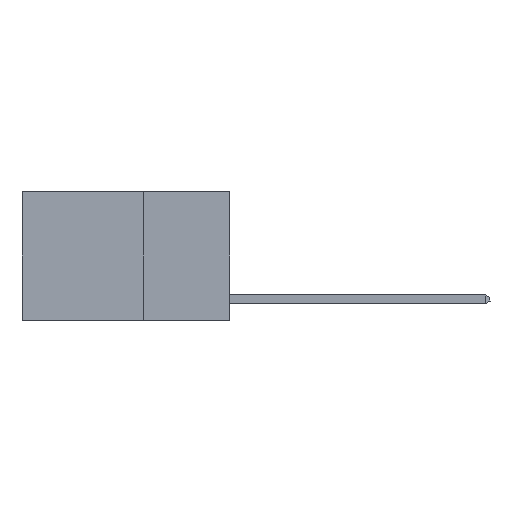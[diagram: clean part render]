
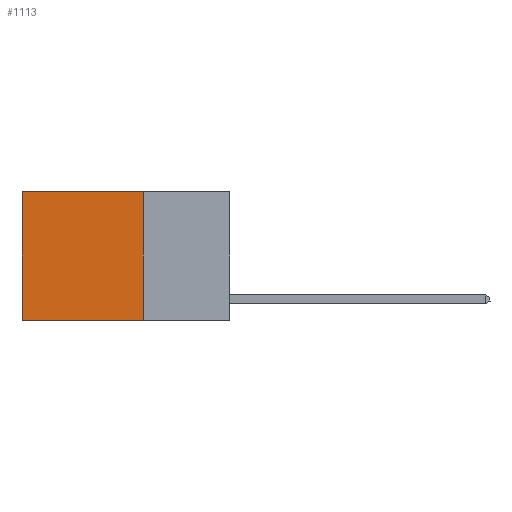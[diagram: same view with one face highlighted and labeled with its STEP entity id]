
A CAD part, left-side view. The second image highlights one B-rep face of the part: STEP entity #1113.
In plain terms, the highlighted planar face has unit normal (-1, 0, 0).
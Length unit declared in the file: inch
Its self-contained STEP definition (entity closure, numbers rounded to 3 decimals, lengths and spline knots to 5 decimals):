
#181 = DIRECTION ( 'NONE',  ( 1., 0., 0. ) ) ;
#607 = CARTESIAN_POINT ( 'NONE',  ( 0.2625, 0.25, -0.37 ) ) ;
#617 = VECTOR ( 'NONE', #15308, 39.37008 ) ;
#680 = CARTESIAN_POINT ( 'NONE',  ( 0.2625, 0.25, 0. ) ) ;
#1113 = ADVANCED_FACE ( 'NONE', ( #6181 ), #6401, .F. ) ;
#1139 = LINE ( 'NONE', #12861, #6908 ) ;
#1286 = VERTEX_POINT ( 'NONE', #11385 ) ;
#1563 = CARTESIAN_POINT ( 'NONE',  ( 0.2625, 0.6, 0. ) ) ;
#1657 = AXIS2_PLACEMENT_3D ( 'NONE', #13498, #181, #7587 ) ;
#2955 = ORIENTED_EDGE ( 'NONE', *, *, #6551, .F. ) ;
#3076 = EDGE_CURVE ( 'NONE', #11134, #11323, #7066, .T. ) ;
#3170 = VECTOR ( 'NONE', #4371, 39.37008 ) ;
#3429 = DIRECTION ( 'NONE',  ( 0., 1., 0. ) ) ;
#4371 = DIRECTION ( 'NONE',  ( 0., 0., -1. ) ) ;
#5027 = EDGE_CURVE ( 'NONE', #10386, #1286, #1139, .T. ) ;
#6181 = FACE_OUTER_BOUND ( 'NONE', #11039, .T. ) ;
#6401 = PLANE ( 'NONE',  #1657 ) ;
#6551 = EDGE_CURVE ( 'NONE', #11323, #1286, #6886, .T. ) ;
#6660 = DIRECTION ( 'NONE',  ( 0., 0., -1. ) ) ;
#6662 = ORIENTED_EDGE ( 'NONE', *, *, #3076, .F. ) ;
#6707 = ORIENTED_EDGE ( 'NONE', *, *, #10562, .T. ) ;
#6886 = LINE ( 'NONE', #7164, #10691 ) ;
#6908 = VECTOR ( 'NONE', #6660, 39.37008 ) ;
#7066 = LINE ( 'NONE', #680, #3170 ) ;
#7164 = CARTESIAN_POINT ( 'NONE',  ( 0.2625, 0.25, -0.37 ) ) ;
#7587 = DIRECTION ( 'NONE',  ( 0., 0., -1. ) ) ;
#9226 = CARTESIAN_POINT ( 'NONE',  ( 0.2625, 0.25, 0. ) ) ;
#10386 = VERTEX_POINT ( 'NONE', #1563 ) ;
#10562 = EDGE_CURVE ( 'NONE', #11134, #10386, #15433, .T. ) ;
#10691 = VECTOR ( 'NONE', #3429, 39.37008 ) ;
#11039 = EDGE_LOOP ( 'NONE', ( #14850, #2955, #6662, #6707 ) ) ;
#11134 = VERTEX_POINT ( 'NONE', #15022 ) ;
#11323 = VERTEX_POINT ( 'NONE', #607 ) ;
#11385 = CARTESIAN_POINT ( 'NONE',  ( 0.2625, 0.6, -0.37 ) ) ;
#12861 = CARTESIAN_POINT ( 'NONE',  ( 0.2625, 0.6, 0. ) ) ;
#13498 = CARTESIAN_POINT ( 'NONE',  ( 0.2625, 0.25, 0. ) ) ;
#14850 = ORIENTED_EDGE ( 'NONE', *, *, #5027, .T. ) ;
#15022 = CARTESIAN_POINT ( 'NONE',  ( 0.2625, 0.25, 0. ) ) ;
#15308 = DIRECTION ( 'NONE',  ( 0., 1., 0. ) ) ;
#15433 = LINE ( 'NONE', #9226, #617 ) ;
